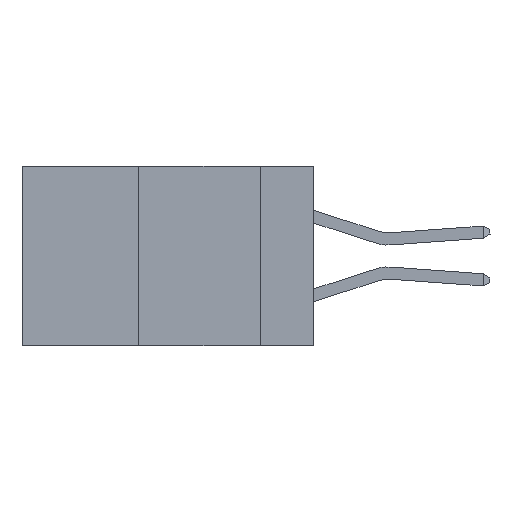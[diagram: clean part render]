
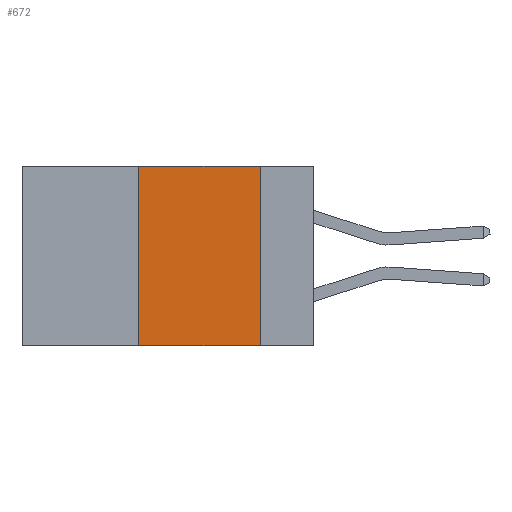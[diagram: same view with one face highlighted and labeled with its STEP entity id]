
A CAD part, left-side view. The second image highlights one B-rep face of the part: STEP entity #672.
In plain terms, the highlighted planar face has unit normal (-1, 0, 0).
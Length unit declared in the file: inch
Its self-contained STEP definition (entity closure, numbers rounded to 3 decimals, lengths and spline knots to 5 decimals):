
#672 = ADVANCED_FACE ( 'NONE', ( #5643 ), #10090, .F. ) ;
#1011 = VECTOR ( 'NONE', #13541, 39.37008 ) ;
#1423 = ORIENTED_EDGE ( 'NONE', *, *, #10677, .F. ) ;
#1797 = ORIENTED_EDGE ( 'NONE', *, *, #15567, .T. ) ;
#1928 = CARTESIAN_POINT ( 'NONE',  ( 0., 0.6, -0.37 ) ) ;
#2340 = LINE ( 'NONE', #1928, #11540 ) ;
#2397 = LINE ( 'NONE', #14683, #14910 ) ;
#2455 = LINE ( 'NONE', #13835, #15360 ) ;
#3771 = DIRECTION ( 'NONE',  ( 0., 0., -1. ) ) ;
#4294 = LINE ( 'NONE', #12262, #1011 ) ;
#5345 = VERTEX_POINT ( 'NONE', #5923 ) ;
#5643 = FACE_OUTER_BOUND ( 'NONE', #10925, .T. ) ;
#5923 = CARTESIAN_POINT ( 'NONE',  ( 0., 0.11, 0. ) ) ;
#6181 = CARTESIAN_POINT ( 'NONE',  ( 0., 0.36, -0.37 ) ) ;
#7485 = EDGE_CURVE ( 'NONE', #5345, #11605, #2455, .T. ) ;
#7869 = CARTESIAN_POINT ( 'NONE',  ( 0., 0.11, -0.37 ) ) ;
#9167 = CARTESIAN_POINT ( 'NONE',  ( 0., 0.6, 0. ) ) ;
#9457 = CARTESIAN_POINT ( 'NONE',  ( 0., 0.36, 0. ) ) ;
#9643 = DIRECTION ( 'NONE',  ( 0., 0., -1. ) ) ;
#9746 = ORIENTED_EDGE ( 'NONE', *, *, #7485, .F. ) ;
#10002 = EDGE_CURVE ( 'NONE', #14269, #10556, #2397, .T. ) ;
#10008 = DIRECTION ( 'NONE',  ( 1., 0., 0. ) ) ;
#10090 = PLANE ( 'NONE',  #13889 ) ;
#10556 = VERTEX_POINT ( 'NONE', #9457 ) ;
#10677 = EDGE_CURVE ( 'NONE', #10556, #5345, #4294, .T. ) ;
#10925 = EDGE_LOOP ( 'NONE', ( #9746, #1423, #14696, #1797 ) ) ;
#10938 = DIRECTION ( 'NONE',  ( 0., 0., 1. ) ) ;
#11540 = VECTOR ( 'NONE', #13260, 39.37008 ) ;
#11605 = VERTEX_POINT ( 'NONE', #7869 ) ;
#12262 = CARTESIAN_POINT ( 'NONE',  ( 0., 0.6, 0. ) ) ;
#13260 = DIRECTION ( 'NONE',  ( 0., -1., 0. ) ) ;
#13541 = DIRECTION ( 'NONE',  ( 0., -1., 0. ) ) ;
#13835 = CARTESIAN_POINT ( 'NONE',  ( 0., 0.11, 0. ) ) ;
#13889 = AXIS2_PLACEMENT_3D ( 'NONE', #9167, #10008, #9643 ) ;
#14269 = VERTEX_POINT ( 'NONE', #6181 ) ;
#14683 = CARTESIAN_POINT ( 'NONE',  ( 0., 0.36, 0. ) ) ;
#14696 = ORIENTED_EDGE ( 'NONE', *, *, #10002, .F. ) ;
#14910 = VECTOR ( 'NONE', #10938, 39.37008 ) ;
#15360 = VECTOR ( 'NONE', #3771, 39.37008 ) ;
#15567 = EDGE_CURVE ( 'NONE', #14269, #11605, #2340, .T. ) ;
